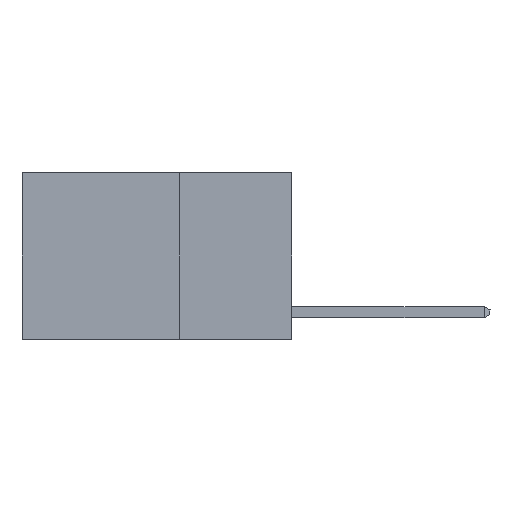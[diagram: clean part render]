
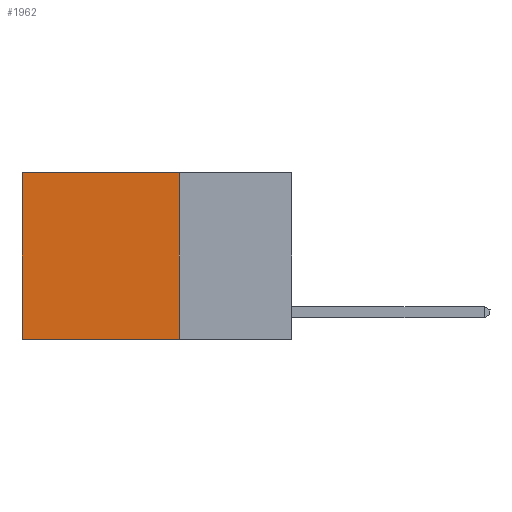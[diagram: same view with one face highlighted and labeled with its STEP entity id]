
A CAD part, left-side view. The second image highlights one B-rep face of the part: STEP entity #1962.
In plain terms, the highlighted planar face has unit normal (-1, 0, 0).
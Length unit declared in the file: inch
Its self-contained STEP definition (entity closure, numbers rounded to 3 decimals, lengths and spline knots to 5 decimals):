
#136 = LINE ( 'NONE', #8828, #12842 ) ;
#302 = CARTESIAN_POINT ( 'NONE',  ( 0.2625, 0.25, -0.37 ) ) ;
#413 = CARTESIAN_POINT ( 'NONE',  ( 0.2625, 0.25, -0.37 ) ) ;
#1594 = ORIENTED_EDGE ( 'NONE', *, *, #7421, .T. ) ;
#1610 = ORIENTED_EDGE ( 'NONE', *, *, #11166, .F. ) ;
#1622 = ORIENTED_EDGE ( 'NONE', *, *, #3059, .F. ) ;
#1649 = ORIENTED_EDGE ( 'NONE', *, *, #9544, .T. ) ;
#1689 = DIRECTION ( 'NONE',  ( 0., 1., 0. ) ) ;
#1962 = ADVANCED_FACE ( 'NONE', ( #3239 ), #12077, .F. ) ;
#2285 = DIRECTION ( 'NONE',  ( 0., 0., -1. ) ) ;
#3059 = EDGE_CURVE ( 'NONE', #3656, #8611, #11231, .T. ) ;
#3239 = FACE_OUTER_BOUND ( 'NONE', #5043, .T. ) ;
#3656 = VERTEX_POINT ( 'NONE', #5072 ) ;
#5043 = EDGE_LOOP ( 'NONE', ( #1594, #1610, #1622, #1649 ) ) ;
#5072 = CARTESIAN_POINT ( 'NONE',  ( 0.2625, 0.25, 0. ) ) ;
#5174 = CARTESIAN_POINT ( 'NONE',  ( 0.2625, 0.25, 0. ) ) ;
#6346 = VERTEX_POINT ( 'NONE', #10697 ) ;
#6477 = DIRECTION ( 'NONE',  ( 0., 1., 0. ) ) ;
#7421 = EDGE_CURVE ( 'NONE', #10497, #6346, #12174, .T. ) ;
#7872 = LINE ( 'NONE', #413, #12795 ) ;
#8611 = VERTEX_POINT ( 'NONE', #302 ) ;
#8828 = CARTESIAN_POINT ( 'NONE',  ( 0.2625, 0.25, 0. ) ) ;
#8968 = VECTOR ( 'NONE', #2285, 39.37008 ) ;
#9544 = EDGE_CURVE ( 'NONE', #3656, #10497, #136, .T. ) ;
#10302 = CARTESIAN_POINT ( 'NONE',  ( 0.2625, 0.6, 0. ) ) ;
#10415 = CARTESIAN_POINT ( 'NONE',  ( 0.2625, 0.6, 0. ) ) ;
#10497 = VERTEX_POINT ( 'NONE', #10302 ) ;
#10697 = CARTESIAN_POINT ( 'NONE',  ( 0.2625, 0.6, -0.37 ) ) ;
#10914 = VECTOR ( 'NONE', #11256, 39.37008 ) ;
#11166 = EDGE_CURVE ( 'NONE', #8611, #6346, #7872, .T. ) ;
#11231 = LINE ( 'NONE', #5174, #10914 ) ;
#11256 = DIRECTION ( 'NONE',  ( 0., 0., -1. ) ) ;
#11712 = AXIS2_PLACEMENT_3D ( 'NONE', #12454, #11915, #11770 ) ;
#11770 = DIRECTION ( 'NONE',  ( 0., 0., -1. ) ) ;
#11915 = DIRECTION ( 'NONE',  ( 1., 0., 0. ) ) ;
#12077 = PLANE ( 'NONE',  #11712 ) ;
#12174 = LINE ( 'NONE', #10415, #8968 ) ;
#12454 = CARTESIAN_POINT ( 'NONE',  ( 0.2625, 0.25, 0. ) ) ;
#12795 = VECTOR ( 'NONE', #6477, 39.37008 ) ;
#12842 = VECTOR ( 'NONE', #1689, 39.37008 ) ;
